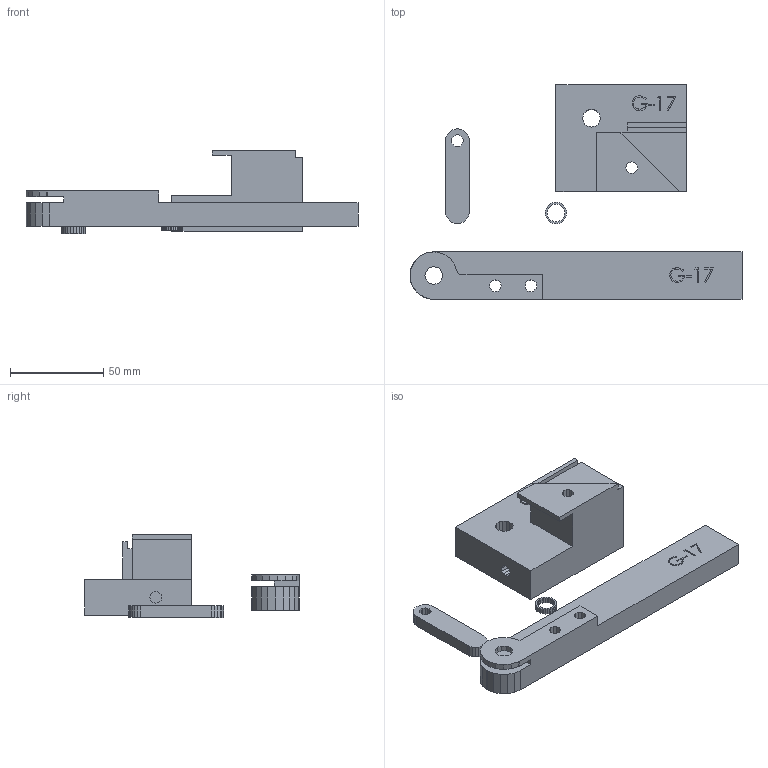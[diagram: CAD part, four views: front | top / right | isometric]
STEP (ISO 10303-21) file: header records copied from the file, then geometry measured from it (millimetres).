
FILE_DESCRIPTION(('STEP AP214'),'1');
FILE_NAME('G17 all parts.stp','2020-03-31T01:17:49',(' '),(' '),'Spatial InterOp 3D',' ',' ');
FILE_SCHEMA(('AUTOMOTIVE_DESIGN { 1 0 10303 214 1 1 1 1 }'));
Length unit declared in the file: metre
Products named in the file (1): Solid
Bounding box: 177.8 x 114.85 x 44.45 mm (x, y, z)
Volume: 167009 mm3; surface area: 38170.4 mm2
Topology: 4 solids, 4 shells, 374 faces, 1085 edges, 728 vertices
Faces by surface type: plane 374
Entity records: 12174 total; most frequent: CARTESIAN_POINT 2191, ORIENTED_EDGE 2170, DIRECTION 1841, EDGE_CURVE 1085, LINE 1085, VECTOR 1085, VERTEX_POINT 728, EDGE_LOOP 399
